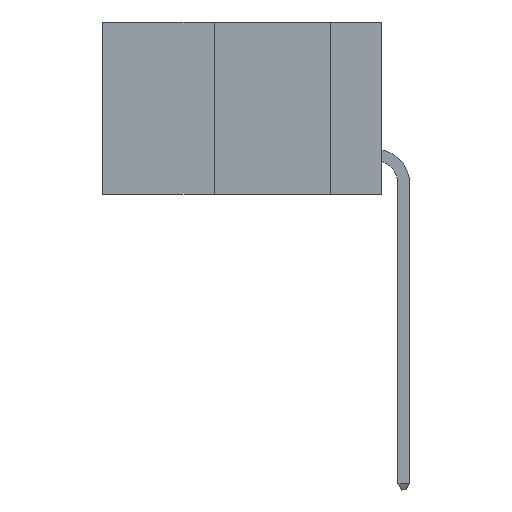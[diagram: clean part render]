
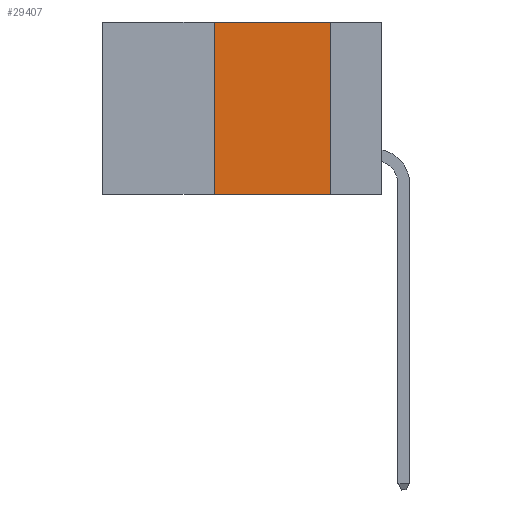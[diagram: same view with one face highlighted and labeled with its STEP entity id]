
A CAD part, left-side view. The second image highlights one B-rep face of the part: STEP entity #29407.
In plain terms, the highlighted planar face has unit normal (-1, 0, 0).
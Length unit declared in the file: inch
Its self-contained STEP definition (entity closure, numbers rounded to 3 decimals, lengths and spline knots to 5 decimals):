
#363 = ORIENTED_EDGE ( 'NONE', *, *, #7669, .F. ) ;
#1160 = VECTOR ( 'NONE', #18068, 39.37008 ) ;
#2050 = ORIENTED_EDGE ( 'NONE', *, *, #41606, .T. ) ;
#2927 = PLANE ( 'NONE',  #7938 ) ;
#3553 = EDGE_CURVE ( 'NONE', #44239, #20161, #34835, .T. ) ;
#3630 = CARTESIAN_POINT ( 'NONE',  ( 0., 0.11, 0. ) ) ;
#6018 = CARTESIAN_POINT ( 'NONE',  ( 0., 0.11, -0.37 ) ) ;
#6070 = VERTEX_POINT ( 'NONE', #34224 ) ;
#7669 = EDGE_CURVE ( 'NONE', #6070, #28171, #46446, .T. ) ;
#7712 = LINE ( 'NONE', #21554, #23658 ) ;
#7938 = AXIS2_PLACEMENT_3D ( 'NONE', #36408, #17991, #14760 ) ;
#8061 = EDGE_LOOP ( 'NONE', ( #30192, #28953, #363, #2050 ) ) ;
#11154 = FACE_OUTER_BOUND ( 'NONE', #8061, .T. ) ;
#14760 = DIRECTION ( 'NONE',  ( 0., 0., -1. ) ) ;
#16476 = CARTESIAN_POINT ( 'NONE',  ( 0., 0.36, 0. ) ) ;
#17485 = EDGE_CURVE ( 'NONE', #28171, #44239, #40151, .T. ) ;
#17991 = DIRECTION ( 'NONE',  ( 1., 0., 0. ) ) ;
#18068 = DIRECTION ( 'NONE',  ( 0., -1., 0. ) ) ;
#19905 = VECTOR ( 'NONE', #33979, 39.37008 ) ;
#20161 = VERTEX_POINT ( 'NONE', #6018 ) ;
#21554 = CARTESIAN_POINT ( 'NONE',  ( 0., 0.6, -0.37 ) ) ;
#23658 = VECTOR ( 'NONE', #46754, 39.37008 ) ;
#25000 = CARTESIAN_POINT ( 'NONE',  ( 0., 0.6, 0. ) ) ;
#28171 = VERTEX_POINT ( 'NONE', #16476 ) ;
#28396 = CARTESIAN_POINT ( 'NONE',  ( 0., 0.36, 0. ) ) ;
#28873 = CARTESIAN_POINT ( 'NONE',  ( 0., 0.11, 0. ) ) ;
#28953 = ORIENTED_EDGE ( 'NONE', *, *, #17485, .F. ) ;
#29407 = ADVANCED_FACE ( 'NONE', ( #11154 ), #2927, .F. ) ;
#30192 = ORIENTED_EDGE ( 'NONE', *, *, #3553, .F. ) ;
#33033 = DIRECTION ( 'NONE',  ( 0., 0., 1. ) ) ;
#33979 = DIRECTION ( 'NONE',  ( 0., 0., -1. ) ) ;
#34224 = CARTESIAN_POINT ( 'NONE',  ( 0., 0.36, -0.37 ) ) ;
#34835 = LINE ( 'NONE', #3630, #19905 ) ;
#36408 = CARTESIAN_POINT ( 'NONE',  ( 0., 0.6, 0. ) ) ;
#40151 = LINE ( 'NONE', #25000, #1160 ) ;
#41606 = EDGE_CURVE ( 'NONE', #6070, #20161, #7712, .T. ) ;
#42459 = VECTOR ( 'NONE', #33033, 39.37008 ) ;
#44239 = VERTEX_POINT ( 'NONE', #28873 ) ;
#46446 = LINE ( 'NONE', #28396, #42459 ) ;
#46754 = DIRECTION ( 'NONE',  ( 0., -1., 0. ) ) ;
